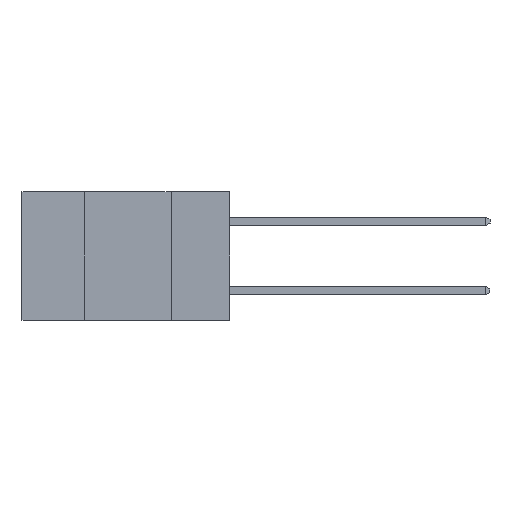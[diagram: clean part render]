
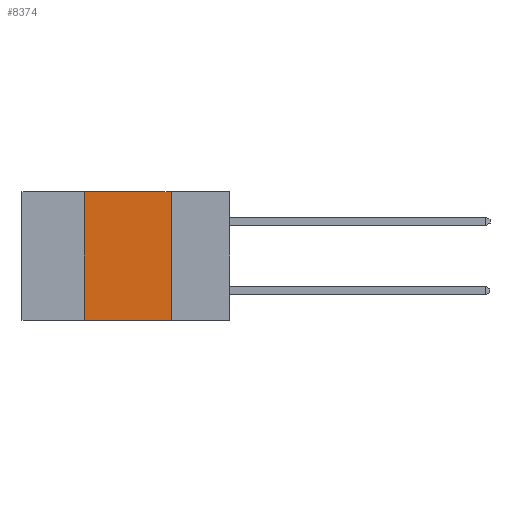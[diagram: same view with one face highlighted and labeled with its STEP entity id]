
A CAD part, left-side view. The second image highlights one B-rep face of the part: STEP entity #8374.
In plain terms, the highlighted planar face has unit normal (-1, 0, 0).
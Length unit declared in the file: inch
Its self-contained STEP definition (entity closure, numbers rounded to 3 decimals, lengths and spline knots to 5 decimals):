
#292 = EDGE_CURVE ( 'NONE', #2147, #1606, #1924, .T. ) ;
#294 = EDGE_CURVE ( 'NONE', #9045, #6940, #4433, .T. ) ;
#297 = EDGE_CURVE ( 'NONE', #9045, #1606, #10275, .T. ) ;
#664 = DIRECTION ( 'NONE',  ( 0., -1., 0. ) ) ;
#1016 = EDGE_LOOP ( 'NONE', ( #4655, #8519, #4510, #8552 ) ) ;
#1413 = CARTESIAN_POINT ( 'NONE',  ( 0., 0.42, 0. ) ) ;
#1606 = VERTEX_POINT ( 'NONE', #6414 ) ;
#1924 = LINE ( 'NONE', #5571, #8313 ) ;
#2147 = VERTEX_POINT ( 'NONE', #6653 ) ;
#2367 = DIRECTION ( 'NONE',  ( 0., 0., -1. ) ) ;
#4150 = VECTOR ( 'NONE', #8983, 39.37008 ) ;
#4429 = CARTESIAN_POINT ( 'NONE',  ( 0., 0.6, 0. ) ) ;
#4433 = LINE ( 'NONE', #6523, #4150 ) ;
#4510 = ORIENTED_EDGE ( 'NONE', *, *, #294, .F. ) ;
#4655 = ORIENTED_EDGE ( 'NONE', *, *, #292, .F. ) ;
#5267 = DIRECTION ( 'NONE',  ( 0., 0., -1. ) ) ;
#5571 = CARTESIAN_POINT ( 'NONE',  ( 0., 0.17, 0. ) ) ;
#5933 = EDGE_CURVE ( 'NONE', #6940, #2147, #6471, .T. ) ;
#6327 = CARTESIAN_POINT ( 'NONE',  ( 0., 0.6, -0.37 ) ) ;
#6414 = CARTESIAN_POINT ( 'NONE',  ( 0., 0.17, -0.37 ) ) ;
#6471 = LINE ( 'NONE', #10528, #10712 ) ;
#6523 = CARTESIAN_POINT ( 'NONE',  ( 0., 0.42, 0. ) ) ;
#6653 = CARTESIAN_POINT ( 'NONE',  ( 0., 0.17, 0. ) ) ;
#6880 = AXIS2_PLACEMENT_3D ( 'NONE', #4429, #9800, #5267 ) ;
#6940 = VERTEX_POINT ( 'NONE', #1413 ) ;
#8067 = VECTOR ( 'NONE', #9365, 39.37008 ) ;
#8313 = VECTOR ( 'NONE', #2367, 39.37008 ) ;
#8374 = ADVANCED_FACE ( 'NONE', ( #10470 ), #9038, .F. ) ;
#8519 = ORIENTED_EDGE ( 'NONE', *, *, #5933, .F. ) ;
#8552 = ORIENTED_EDGE ( 'NONE', *, *, #297, .T. ) ;
#8596 = CARTESIAN_POINT ( 'NONE',  ( 0., 0.42, -0.37 ) ) ;
#8983 = DIRECTION ( 'NONE',  ( 0., 0., 1. ) ) ;
#9038 = PLANE ( 'NONE',  #6880 ) ;
#9045 = VERTEX_POINT ( 'NONE', #8596 ) ;
#9365 = DIRECTION ( 'NONE',  ( 0., -1., 0. ) ) ;
#9800 = DIRECTION ( 'NONE',  ( 1., 0., 0. ) ) ;
#10275 = LINE ( 'NONE', #6327, #8067 ) ;
#10470 = FACE_OUTER_BOUND ( 'NONE', #1016, .T. ) ;
#10528 = CARTESIAN_POINT ( 'NONE',  ( 0., 0.6, 0. ) ) ;
#10712 = VECTOR ( 'NONE', #664, 39.37008 ) ;
